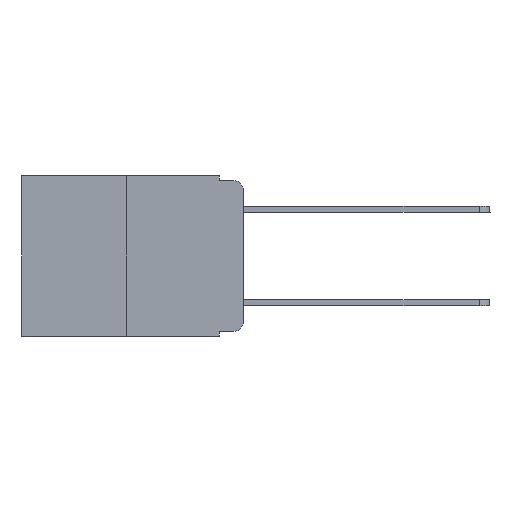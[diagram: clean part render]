
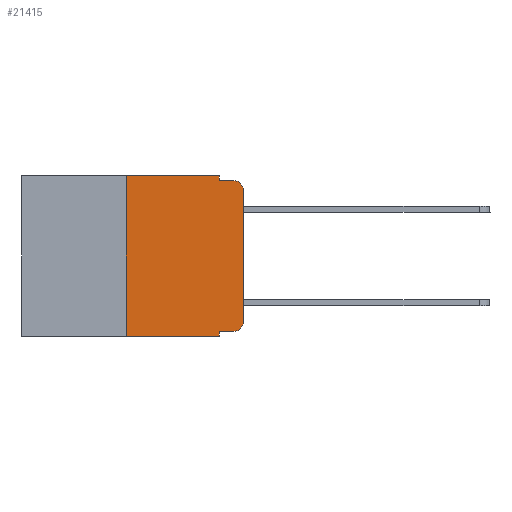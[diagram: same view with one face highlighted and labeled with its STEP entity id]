
A CAD part, left-side view. The second image highlights one B-rep face of the part: STEP entity #21415.
In plain terms, the highlighted planar face has unit normal (-1, 0, 0).
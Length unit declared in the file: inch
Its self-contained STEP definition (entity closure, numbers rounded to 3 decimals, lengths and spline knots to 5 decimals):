
#80 = VERTEX_POINT ( 'NONE', #1001 ) ;
#621 = LINE ( 'NONE', #3148, #19957 ) ;
#883 = CARTESIAN_POINT ( 'NONE',  ( 0., 0.02, -0.313 ) ) ;
#989 = DIRECTION ( 'NONE',  ( 1., 0., 0. ) ) ;
#1001 = CARTESIAN_POINT ( 'NONE',  ( 0., 0.25, -0.343 ) ) ;
#1214 = DIRECTION ( 'NONE',  ( 0., 0., -1. ) ) ;
#1924 = EDGE_CURVE ( 'NONE', #24170, #22052, #18888, .T. ) ;
#2240 = EDGE_CURVE ( 'NONE', #12790, #21742, #10065, .T. ) ;
#2399 = DIRECTION ( 'NONE',  ( 0., -1., 0. ) ) ;
#2448 = CARTESIAN_POINT ( 'NONE',  ( 0., 0.02, -0.03 ) ) ;
#2528 = LINE ( 'NONE', #14717, #15755 ) ;
#2706 = CARTESIAN_POINT ( 'NONE',  ( 0., 0.473, 0. ) ) ;
#3148 = CARTESIAN_POINT ( 'NONE',  ( 0., 0.25, 0. ) ) ;
#3223 = EDGE_CURVE ( 'NONE', #24170, #3239, #16490, .T. ) ;
#3239 = VERTEX_POINT ( 'NONE', #23663 ) ;
#3361 = CARTESIAN_POINT ( 'NONE',  ( 0., 0.051, 0. ) ) ;
#3491 = ORIENTED_EDGE ( 'NONE', *, *, #20271, .F. ) ;
#4221 = LINE ( 'NONE', #3361, #8041 ) ;
#4720 = DIRECTION ( 'NONE',  ( 0., 0., -1. ) ) ;
#4728 = VERTEX_POINT ( 'NONE', #15121 ) ;
#5056 = VECTOR ( 'NONE', #15876, 39.37008 ) ;
#5532 = EDGE_LOOP ( 'NONE', ( #14069, #6940, #11839, #3491, #15810, #11078, #19418, #20215, #18838, #15174 ) ) ;
#5996 = CARTESIAN_POINT ( 'NONE',  ( 0., 0.473, -0.343 ) ) ;
#6220 = EDGE_CURVE ( 'NONE', #14325, #8478, #2528, .T. ) ;
#6262 = VECTOR ( 'NONE', #13525, 39.37008 ) ;
#6537 = DIRECTION ( 'NONE',  ( 0., 0., -1. ) ) ;
#6651 = EDGE_CURVE ( 'NONE', #4728, #7412, #16024, .T. ) ;
#6819 = AXIS2_PLACEMENT_3D ( 'NONE', #2448, #19662, #6537 ) ;
#6940 = ORIENTED_EDGE ( 'NONE', *, *, #7967, .T. ) ;
#7293 = DIRECTION ( 'NONE',  ( 0., -1., 0. ) ) ;
#7412 = VERTEX_POINT ( 'NONE', #8676 ) ;
#7967 = EDGE_CURVE ( 'NONE', #8478, #7412, #23096, .T. ) ;
#8041 = VECTOR ( 'NONE', #24057, 39.37008 ) ;
#8394 = EDGE_CURVE ( 'NONE', #80, #3239, #11316, .T. ) ;
#8478 = VERTEX_POINT ( 'NONE', #9850 ) ;
#8676 = CARTESIAN_POINT ( 'NONE',  ( 0., 0.02, -0.01 ) ) ;
#9104 = CARTESIAN_POINT ( 'NONE',  ( 0., 0.051, -0.333 ) ) ;
#9582 = DIRECTION ( 'NONE',  ( 0., 0., 1. ) ) ;
#9850 = CARTESIAN_POINT ( 'NONE',  ( 0., 0., -0.03 ) ) ;
#10065 = LINE ( 'NONE', #2706, #5056 ) ;
#10174 = CARTESIAN_POINT ( 'NONE',  ( 0., 0.051, -0.333 ) ) ;
#10245 = PLANE ( 'NONE',  #10941 ) ;
#10941 = AXIS2_PLACEMENT_3D ( 'NONE', #12170, #989, #4720 ) ;
#11078 = ORIENTED_EDGE ( 'NONE', *, *, #12894, .F. ) ;
#11316 = LINE ( 'NONE', #5996, #16352 ) ;
#11839 = ORIENTED_EDGE ( 'NONE', *, *, #6651, .F. ) ;
#12170 = CARTESIAN_POINT ( 'NONE',  ( 0., 0.473, 0. ) ) ;
#12401 = CARTESIAN_POINT ( 'NONE',  ( 0., 0.051, 0. ) ) ;
#12790 = VERTEX_POINT ( 'NONE', #14955 ) ;
#12894 = EDGE_CURVE ( 'NONE', #80, #12790, #621, .T. ) ;
#12930 = VECTOR ( 'NONE', #1214, 39.37008 ) ;
#13525 = DIRECTION ( 'NONE',  ( 0., -1., 0. ) ) ;
#14069 = ORIENTED_EDGE ( 'NONE', *, *, #6220, .T. ) ;
#14077 = DIRECTION ( 'NONE',  ( 0., 0., 1. ) ) ;
#14325 = VERTEX_POINT ( 'NONE', #23898 ) ;
#14717 = CARTESIAN_POINT ( 'NONE',  ( 0., 0., 0. ) ) ;
#14955 = CARTESIAN_POINT ( 'NONE',  ( 0., 0.25, 0. ) ) ;
#15121 = CARTESIAN_POINT ( 'NONE',  ( 0., 0.051, -0.01 ) ) ;
#15174 = ORIENTED_EDGE ( 'NONE', *, *, #16563, .T. ) ;
#15645 = FACE_OUTER_BOUND ( 'NONE', #5532, .T. ) ;
#15755 = VECTOR ( 'NONE', #9582, 39.37008 ) ;
#15810 = ORIENTED_EDGE ( 'NONE', *, *, #2240, .F. ) ;
#15876 = DIRECTION ( 'NONE',  ( 0., -1., 0. ) ) ;
#16024 = LINE ( 'NONE', #22200, #16321 ) ;
#16321 = VECTOR ( 'NONE', #7293, 39.37008 ) ;
#16352 = VECTOR ( 'NONE', #2399, 39.37008 ) ;
#16490 = LINE ( 'NONE', #12401, #12930 ) ;
#16563 = EDGE_CURVE ( 'NONE', #22052, #14325, #21520, .T. ) ;
#16874 = AXIS2_PLACEMENT_3D ( 'NONE', #883, #17765, #17845 ) ;
#17765 = DIRECTION ( 'NONE',  ( -1., 0., 0. ) ) ;
#17845 = DIRECTION ( 'NONE',  ( 0., 0., -1. ) ) ;
#18800 = CARTESIAN_POINT ( 'NONE',  ( 0., 0.02, -0.333 ) ) ;
#18838 = ORIENTED_EDGE ( 'NONE', *, *, #1924, .T. ) ;
#18888 = LINE ( 'NONE', #9104, #6262 ) ;
#19418 = ORIENTED_EDGE ( 'NONE', *, *, #8394, .T. ) ;
#19662 = DIRECTION ( 'NONE',  ( -1., 0., 0. ) ) ;
#19957 = VECTOR ( 'NONE', #14077, 39.37008 ) ;
#20215 = ORIENTED_EDGE ( 'NONE', *, *, #3223, .F. ) ;
#20271 = EDGE_CURVE ( 'NONE', #21742, #4728, #4221, .T. ) ;
#21415 = ADVANCED_FACE ( 'NONE', ( #15645 ), #10245, .F. ) ;
#21520 = CIRCLE ( 'NONE', #16874, 0.02 ) ;
#21742 = VERTEX_POINT ( 'NONE', #23555 ) ;
#22052 = VERTEX_POINT ( 'NONE', #18800 ) ;
#22200 = CARTESIAN_POINT ( 'NONE',  ( 0., 0.051, -0.01 ) ) ;
#23096 = CIRCLE ( 'NONE', #6819, 0.02 ) ;
#23555 = CARTESIAN_POINT ( 'NONE',  ( 0., 0.051, 0. ) ) ;
#23663 = CARTESIAN_POINT ( 'NONE',  ( 0., 0.051, -0.343 ) ) ;
#23898 = CARTESIAN_POINT ( 'NONE',  ( 0., 0., -0.313 ) ) ;
#24057 = DIRECTION ( 'NONE',  ( 0., 0., -1. ) ) ;
#24170 = VERTEX_POINT ( 'NONE', #10174 ) ;
